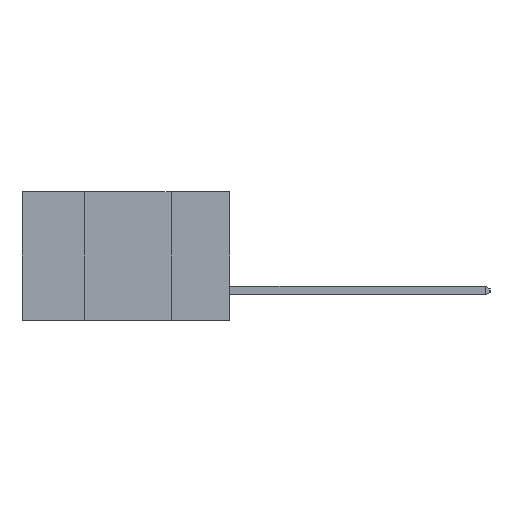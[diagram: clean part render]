
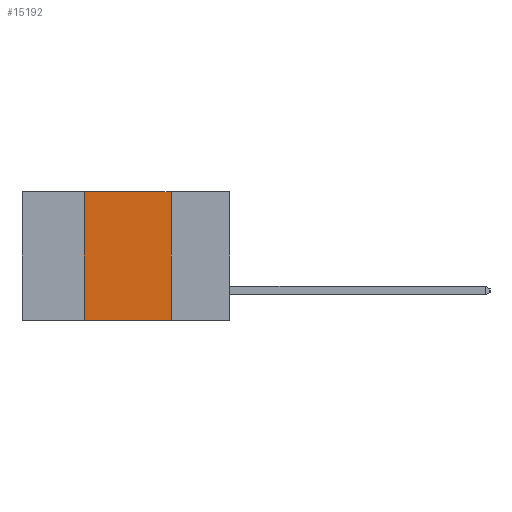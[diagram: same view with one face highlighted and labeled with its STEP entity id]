
A CAD part, left-side view. The second image highlights one B-rep face of the part: STEP entity #15192.
In plain terms, the highlighted planar face has unit normal (-1, 0, 0).
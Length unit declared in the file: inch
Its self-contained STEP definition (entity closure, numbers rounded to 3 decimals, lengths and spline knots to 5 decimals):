
#213 = EDGE_CURVE ( 'NONE', #7332, #10366, #5855, .T. ) ;
#439 = CARTESIAN_POINT ( 'NONE',  ( 0., 0.42, -0.37 ) ) ;
#442 = EDGE_CURVE ( 'NONE', #8221, #1292, #8188, .T. ) ;
#916 = ORIENTED_EDGE ( 'NONE', *, *, #442, .F. ) ;
#1292 = VERTEX_POINT ( 'NONE', #8298 ) ;
#1373 = PLANE ( 'NONE',  #8493 ) ;
#1563 = ORIENTED_EDGE ( 'NONE', *, *, #10169, .F. ) ;
#2097 = DIRECTION ( 'NONE',  ( 0., -1., 0. ) ) ;
#2318 = CARTESIAN_POINT ( 'NONE',  ( 0., 0.17, 0. ) ) ;
#2716 = CARTESIAN_POINT ( 'NONE',  ( 0., 0.6, 0. ) ) ;
#4013 = DIRECTION ( 'NONE',  ( 1., 0., 0. ) ) ;
#4021 = CARTESIAN_POINT ( 'NONE',  ( 0., 0.42, 0. ) ) ;
#4957 = ORIENTED_EDGE ( 'NONE', *, *, #5288, .T. ) ;
#5074 = VECTOR ( 'NONE', #10245, 39.37008 ) ;
#5288 = EDGE_CURVE ( 'NONE', #7332, #1292, #12899, .T. ) ;
#5315 = DIRECTION ( 'NONE',  ( 0., 0., -1. ) ) ;
#5555 = CARTESIAN_POINT ( 'NONE',  ( 0., 0.6, -0.37 ) ) ;
#5855 = LINE ( 'NONE', #12529, #5074 ) ;
#6005 = EDGE_LOOP ( 'NONE', ( #916, #1563, #8282, #4957 ) ) ;
#6277 = VECTOR ( 'NONE', #13016, 39.37008 ) ;
#7332 = VERTEX_POINT ( 'NONE', #439 ) ;
#7773 = LINE ( 'NONE', #10948, #13982 ) ;
#8188 = LINE ( 'NONE', #10513, #15176 ) ;
#8221 = VERTEX_POINT ( 'NONE', #2318 ) ;
#8282 = ORIENTED_EDGE ( 'NONE', *, *, #213, .F. ) ;
#8298 = CARTESIAN_POINT ( 'NONE',  ( 0., 0.17, -0.37 ) ) ;
#8493 = AXIS2_PLACEMENT_3D ( 'NONE', #2716, #4013, #12762 ) ;
#10078 = FACE_OUTER_BOUND ( 'NONE', #6005, .T. ) ;
#10169 = EDGE_CURVE ( 'NONE', #10366, #8221, #7773, .T. ) ;
#10245 = DIRECTION ( 'NONE',  ( 0., 0., 1. ) ) ;
#10366 = VERTEX_POINT ( 'NONE', #4021 ) ;
#10513 = CARTESIAN_POINT ( 'NONE',  ( 0., 0.17, 0. ) ) ;
#10948 = CARTESIAN_POINT ( 'NONE',  ( 0., 0.6, 0. ) ) ;
#12529 = CARTESIAN_POINT ( 'NONE',  ( 0., 0.42, 0. ) ) ;
#12762 = DIRECTION ( 'NONE',  ( 0., 0., -1. ) ) ;
#12899 = LINE ( 'NONE', #5555, #6277 ) ;
#13016 = DIRECTION ( 'NONE',  ( 0., -1., 0. ) ) ;
#13982 = VECTOR ( 'NONE', #2097, 39.37008 ) ;
#15176 = VECTOR ( 'NONE', #5315, 39.37008 ) ;
#15192 = ADVANCED_FACE ( 'NONE', ( #10078 ), #1373, .F. ) ;
